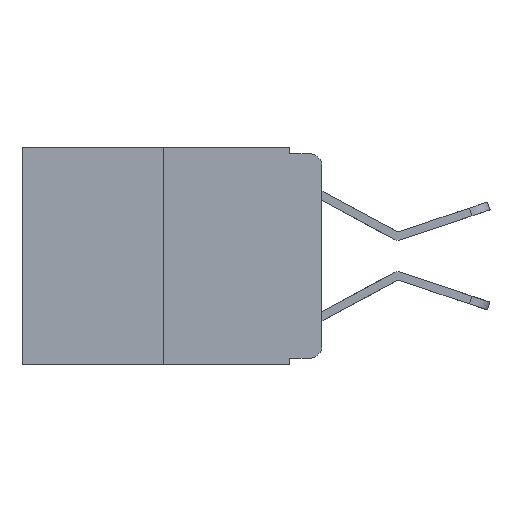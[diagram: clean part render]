
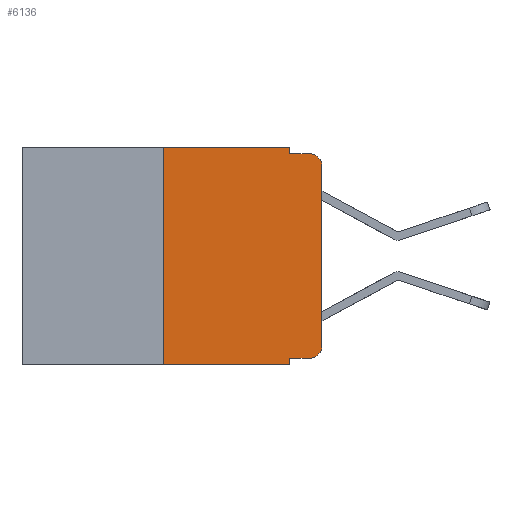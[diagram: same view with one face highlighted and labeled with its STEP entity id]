
A CAD part, left-side view. The second image highlights one B-rep face of the part: STEP entity #6136.
In plain terms, the highlighted planar face has unit normal (-1, 0, 0).
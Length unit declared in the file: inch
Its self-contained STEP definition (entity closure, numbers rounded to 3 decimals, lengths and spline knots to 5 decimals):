
#16 = CARTESIAN_POINT ( 'NONE',  ( 0., 0., 0. ) ) ;
#203 = CARTESIAN_POINT ( 'NONE',  ( 0., 0.02, -0.03 ) ) ;
#225 = VECTOR ( 'NONE', #5143, 39.37008 ) ;
#328 = VERTEX_POINT ( 'NONE', #6553 ) ;
#492 = CIRCLE ( 'NONE', #17942, 0.02 ) ;
#969 = FACE_OUTER_BOUND ( 'NONE', #11617, .T. ) ;
#1212 = CARTESIAN_POINT ( 'NONE',  ( 0., 0.051, -0.01 ) ) ;
#1459 = VERTEX_POINT ( 'NONE', #12672 ) ;
#1615 = CARTESIAN_POINT ( 'NONE',  ( 0., 0.25, 0. ) ) ;
#1653 = DIRECTION ( 'NONE',  ( 0., 0., -1. ) ) ;
#1732 = EDGE_CURVE ( 'NONE', #15802, #1459, #4308, .T. ) ;
#1855 = CARTESIAN_POINT ( 'NONE',  ( 0., 0.25, -0.343 ) ) ;
#1890 = ORIENTED_EDGE ( 'NONE', *, *, #13786, .F. ) ;
#3472 = LINE ( 'NONE', #17023, #10730 ) ;
#3849 = VECTOR ( 'NONE', #9906, 39.37008 ) ;
#4008 = LINE ( 'NONE', #14352, #15087 ) ;
#4277 = DIRECTION ( 'NONE',  ( 0., -1., 0. ) ) ;
#4283 = VECTOR ( 'NONE', #17823, 39.37008 ) ;
#4308 = LINE ( 'NONE', #16, #3849 ) ;
#4752 = LINE ( 'NONE', #14930, #4283 ) ;
#4835 = ORIENTED_EDGE ( 'NONE', *, *, #8935, .T. ) ;
#4915 = AXIS2_PLACEMENT_3D ( 'NONE', #203, #10363, #1653 ) ;
#5113 = ORIENTED_EDGE ( 'NONE', *, *, #12816, .F. ) ;
#5138 = AXIS2_PLACEMENT_3D ( 'NONE', #6245, #16340, #7708 ) ;
#5143 = DIRECTION ( 'NONE',  ( 0., 0., 1. ) ) ;
#5331 = VERTEX_POINT ( 'NONE', #1212 ) ;
#6136 = ADVANCED_FACE ( 'NONE', ( #969 ), #14872, .F. ) ;
#6245 = CARTESIAN_POINT ( 'NONE',  ( 0., 0.473, 0. ) ) ;
#6429 = EDGE_CURVE ( 'NONE', #14370, #15106, #10967, .T. ) ;
#6553 = CARTESIAN_POINT ( 'NONE',  ( 0., 0.02, -0.01 ) ) ;
#6731 = ORIENTED_EDGE ( 'NONE', *, *, #1732, .T. ) ;
#6823 = ORIENTED_EDGE ( 'NONE', *, *, #10873, .F. ) ;
#7012 = EDGE_CURVE ( 'NONE', #15025, #15802, #492, .T. ) ;
#7304 = DIRECTION ( 'NONE',  ( -1., 0., 0. ) ) ;
#7469 = ORIENTED_EDGE ( 'NONE', *, *, #15686, .F. ) ;
#7708 = DIRECTION ( 'NONE',  ( 0., 0., -1. ) ) ;
#7891 = ORIENTED_EDGE ( 'NONE', *, *, #6429, .F. ) ;
#8825 = EDGE_CURVE ( 'NONE', #17925, #13893, #4752, .T. ) ;
#8884 = CARTESIAN_POINT ( 'NONE',  ( 0., 0.473, 0. ) ) ;
#8935 = EDGE_CURVE ( 'NONE', #12166, #15025, #10127, .T. ) ;
#9038 = DIRECTION ( 'NONE',  ( 0., 0., -1. ) ) ;
#9281 = CARTESIAN_POINT ( 'NONE',  ( 0., 0.051, -0.343 ) ) ;
#9856 = DIRECTION ( 'NONE',  ( 0., 0., -1. ) ) ;
#9906 = DIRECTION ( 'NONE',  ( 0., 0., 1. ) ) ;
#9971 = LINE ( 'NONE', #17588, #17171 ) ;
#10127 = LINE ( 'NONE', #13826, #17785 ) ;
#10272 = DIRECTION ( 'NONE',  ( 0., -1., 0. ) ) ;
#10363 = DIRECTION ( 'NONE',  ( -1., 0., 0. ) ) ;
#10730 = VECTOR ( 'NONE', #9856, 39.37008 ) ;
#10873 = EDGE_CURVE ( 'NONE', #12166, #13893, #3472, .T. ) ;
#10919 = DIRECTION ( 'NONE',  ( 0., -1., 0. ) ) ;
#10967 = LINE ( 'NONE', #8884, #11405 ) ;
#11405 = VECTOR ( 'NONE', #10272, 39.37008 ) ;
#11617 = EDGE_LOOP ( 'NONE', ( #6731, #13087, #7469, #1890, #7891, #5113, #15940, #6823, #4835, #15880 ) ) ;
#11642 = CARTESIAN_POINT ( 'NONE',  ( 0., 0.051, 0. ) ) ;
#12166 = VERTEX_POINT ( 'NONE', #18206 ) ;
#12672 = CARTESIAN_POINT ( 'NONE',  ( 0., 0., -0.03 ) ) ;
#12816 = EDGE_CURVE ( 'NONE', #17925, #14370, #15172, .T. ) ;
#13087 = ORIENTED_EDGE ( 'NONE', *, *, #17615, .T. ) ;
#13208 = CARTESIAN_POINT ( 'NONE',  ( 0., 0., -0.313 ) ) ;
#13786 = EDGE_CURVE ( 'NONE', #15106, #5331, #9971, .T. ) ;
#13826 = CARTESIAN_POINT ( 'NONE',  ( 0., 0.051, -0.333 ) ) ;
#13893 = VERTEX_POINT ( 'NONE', #9281 ) ;
#14352 = CARTESIAN_POINT ( 'NONE',  ( 0., 0.051, -0.01 ) ) ;
#14370 = VERTEX_POINT ( 'NONE', #1615 ) ;
#14872 = PLANE ( 'NONE',  #5138 ) ;
#14930 = CARTESIAN_POINT ( 'NONE',  ( 0., 0.473, -0.343 ) ) ;
#15025 = VERTEX_POINT ( 'NONE', #17246 ) ;
#15087 = VECTOR ( 'NONE', #4277, 39.37008 ) ;
#15106 = VERTEX_POINT ( 'NONE', #11642 ) ;
#15172 = LINE ( 'NONE', #15222, #225 ) ;
#15222 = CARTESIAN_POINT ( 'NONE',  ( 0., 0.25, 0. ) ) ;
#15686 = EDGE_CURVE ( 'NONE', #5331, #328, #4008, .T. ) ;
#15802 = VERTEX_POINT ( 'NONE', #13208 ) ;
#15880 = ORIENTED_EDGE ( 'NONE', *, *, #7012, .T. ) ;
#15908 = CARTESIAN_POINT ( 'NONE',  ( 0., 0.02, -0.313 ) ) ;
#15940 = ORIENTED_EDGE ( 'NONE', *, *, #8825, .T. ) ;
#16340 = DIRECTION ( 'NONE',  ( 1., 0., 0. ) ) ;
#17023 = CARTESIAN_POINT ( 'NONE',  ( 0., 0.051, 0. ) ) ;
#17050 = CIRCLE ( 'NONE', #4915, 0.02 ) ;
#17171 = VECTOR ( 'NONE', #9038, 39.37008 ) ;
#17246 = CARTESIAN_POINT ( 'NONE',  ( 0., 0.02, -0.333 ) ) ;
#17356 = DIRECTION ( 'NONE',  ( 0., 0., -1. ) ) ;
#17588 = CARTESIAN_POINT ( 'NONE',  ( 0., 0.051, 0. ) ) ;
#17615 = EDGE_CURVE ( 'NONE', #1459, #328, #17050, .T. ) ;
#17785 = VECTOR ( 'NONE', #10919, 39.37008 ) ;
#17823 = DIRECTION ( 'NONE',  ( 0., -1., 0. ) ) ;
#17925 = VERTEX_POINT ( 'NONE', #1855 ) ;
#17942 = AXIS2_PLACEMENT_3D ( 'NONE', #15908, #7304, #17356 ) ;
#18206 = CARTESIAN_POINT ( 'NONE',  ( 0., 0.051, -0.333 ) ) ;
